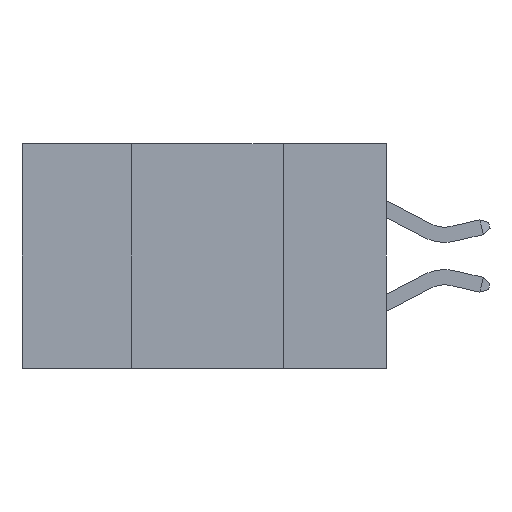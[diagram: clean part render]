
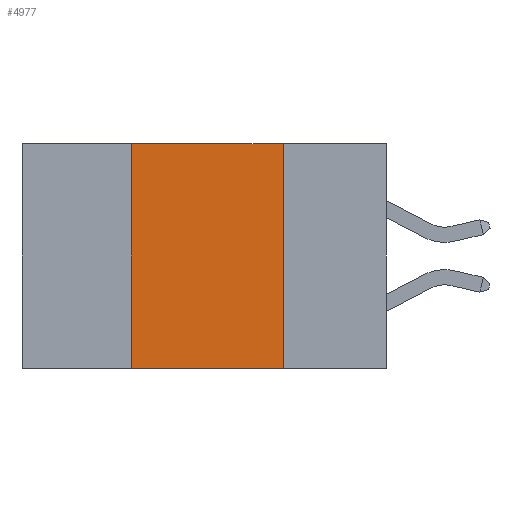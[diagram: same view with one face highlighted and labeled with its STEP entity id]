
A CAD part, left-side view. The second image highlights one B-rep face of the part: STEP entity #4977.
In plain terms, the highlighted planar face has unit normal (-1, 0, 0).
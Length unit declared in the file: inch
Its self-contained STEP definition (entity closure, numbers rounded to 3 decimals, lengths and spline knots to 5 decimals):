
#270 = CARTESIAN_POINT ( 'NONE',  ( 0., 0.42, -0.37 ) ) ;
#289 = VERTEX_POINT ( 'NONE', #8279 ) ;
#295 = DIRECTION ( 'NONE',  ( 0., 0., -1. ) ) ;
#716 = CARTESIAN_POINT ( 'NONE',  ( 0., 0.42, 0. ) ) ;
#1249 = ORIENTED_EDGE ( 'NONE', *, *, #3983, .T. ) ;
#1366 = VECTOR ( 'NONE', #2519, 39.37008 ) ;
#1387 = VECTOR ( 'NONE', #1666, 39.37008 ) ;
#1472 = EDGE_LOOP ( 'NONE', ( #1598, #11983, #12025, #1249 ) ) ;
#1476 = AXIS2_PLACEMENT_3D ( 'NONE', #11646, #1905, #3934 ) ;
#1598 = ORIENTED_EDGE ( 'NONE', *, *, #6361, .F. ) ;
#1666 = DIRECTION ( 'NONE',  ( 0., -1., 0. ) ) ;
#1850 = PLANE ( 'NONE',  #1476 ) ;
#1905 = DIRECTION ( 'NONE',  ( 1., 0., 0. ) ) ;
#2519 = DIRECTION ( 'NONE',  ( 0., 0., 1. ) ) ;
#2787 = FACE_OUTER_BOUND ( 'NONE', #1472, .T. ) ;
#2793 = DIRECTION ( 'NONE',  ( 0., -1., 0. ) ) ;
#3934 = DIRECTION ( 'NONE',  ( 0., 0., -1. ) ) ;
#3983 = EDGE_CURVE ( 'NONE', #11438, #4576, #5645, .T. ) ;
#4072 = LINE ( 'NONE', #4186, #6916 ) ;
#4186 = CARTESIAN_POINT ( 'NONE',  ( 0., 0.17, -0.37 ) ) ;
#4324 = EDGE_CURVE ( 'NONE', #9535, #289, #11393, .T. ) ;
#4504 = CARTESIAN_POINT ( 'NONE',  ( 0., 0.42, -0.37 ) ) ;
#4572 = CARTESIAN_POINT ( 'NONE',  ( 0., 0.6, 0. ) ) ;
#4576 = VERTEX_POINT ( 'NONE', #9806 ) ;
#4717 = CARTESIAN_POINT ( 'NONE',  ( 0., 0.6, -0.37 ) ) ;
#4977 = ADVANCED_FACE ( 'NONE', ( #2787 ), #1850, .F. ) ;
#5645 = LINE ( 'NONE', #4717, #8267 ) ;
#6361 = EDGE_CURVE ( 'NONE', #289, #4576, #4072, .T. ) ;
#6916 = VECTOR ( 'NONE', #295, 39.37008 ) ;
#8267 = VECTOR ( 'NONE', #2793, 39.37008 ) ;
#8279 = CARTESIAN_POINT ( 'NONE',  ( 0., 0.17, 0. ) ) ;
#9113 = EDGE_CURVE ( 'NONE', #11438, #9535, #12145, .T. ) ;
#9535 = VERTEX_POINT ( 'NONE', #716 ) ;
#9806 = CARTESIAN_POINT ( 'NONE',  ( 0., 0.17, -0.37 ) ) ;
#11393 = LINE ( 'NONE', #4572, #1387 ) ;
#11438 = VERTEX_POINT ( 'NONE', #270 ) ;
#11646 = CARTESIAN_POINT ( 'NONE',  ( 0., 0.6, 0. ) ) ;
#11983 = ORIENTED_EDGE ( 'NONE', *, *, #4324, .F. ) ;
#12025 = ORIENTED_EDGE ( 'NONE', *, *, #9113, .F. ) ;
#12145 = LINE ( 'NONE', #4504, #1366 ) ;
